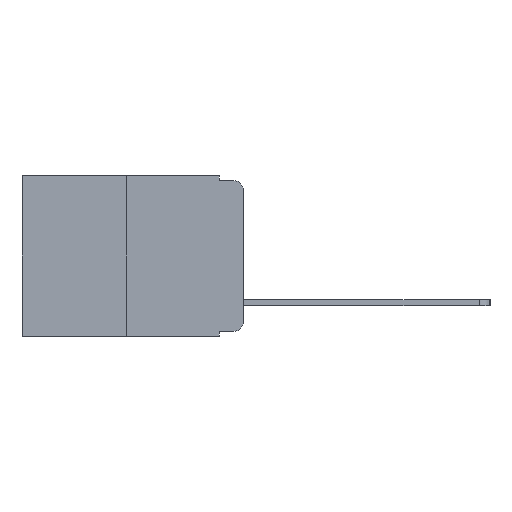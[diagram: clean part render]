
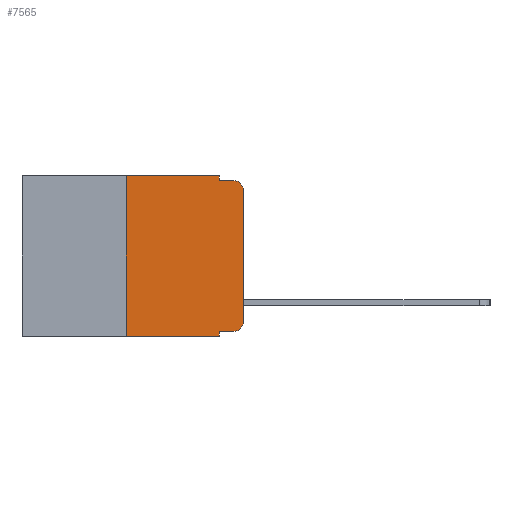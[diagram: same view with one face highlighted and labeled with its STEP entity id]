
A CAD part, left-side view. The second image highlights one B-rep face of the part: STEP entity #7565.
In plain terms, the highlighted planar face has unit normal (-1, 0, 0).
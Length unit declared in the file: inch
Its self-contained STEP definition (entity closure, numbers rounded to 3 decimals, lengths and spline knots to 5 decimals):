
#342 = PLANE ( 'NONE',  #7689 ) ;
#438 = CARTESIAN_POINT ( 'NONE',  ( 0., 0., -0.313 ) ) ;
#507 = LINE ( 'NONE', #7351, #3532 ) ;
#577 = CARTESIAN_POINT ( 'NONE',  ( 0., 0.02, -0.01 ) ) ;
#859 = LINE ( 'NONE', #7053, #8654 ) ;
#865 = CIRCLE ( 'NONE', #8322, 0.02 ) ;
#1341 = VERTEX_POINT ( 'NONE', #12617 ) ;
#1440 = LINE ( 'NONE', #11873, #6818 ) ;
#1530 = DIRECTION ( 'NONE',  ( 0., 0., -1. ) ) ;
#1536 = VERTEX_POINT ( 'NONE', #438 ) ;
#1583 = LINE ( 'NONE', #5567, #4167 ) ;
#1951 = CARTESIAN_POINT ( 'NONE',  ( 0., 0.25, 0. ) ) ;
#2065 = EDGE_CURVE ( 'NONE', #2365, #6524, #12882, .T. ) ;
#2129 = LINE ( 'NONE', #8547, #4656 ) ;
#2168 = DIRECTION ( 'NONE',  ( 0., 0., 1. ) ) ;
#2224 = EDGE_CURVE ( 'NONE', #4842, #2365, #507, .T. ) ;
#2331 = DIRECTION ( 'NONE',  ( -1., 0., 0. ) ) ;
#2365 = VERTEX_POINT ( 'NONE', #1951 ) ;
#2588 = CARTESIAN_POINT ( 'NONE',  ( 0., 0.02, -0.03 ) ) ;
#2692 = EDGE_CURVE ( 'NONE', #1341, #4808, #1440, .T. ) ;
#2743 = ORIENTED_EDGE ( 'NONE', *, *, #9179, .F. ) ;
#2858 = VERTEX_POINT ( 'NONE', #11105 ) ;
#3422 = EDGE_CURVE ( 'NONE', #11238, #4808, #865, .T. ) ;
#3443 = ORIENTED_EDGE ( 'NONE', *, *, #9512, .T. ) ;
#3532 = VECTOR ( 'NONE', #2168, 39.37008 ) ;
#3557 = CARTESIAN_POINT ( 'NONE',  ( 0., 0.051, -0.333 ) ) ;
#3721 = CARTESIAN_POINT ( 'NONE',  ( 0., 0.473, 0. ) ) ;
#3861 = CARTESIAN_POINT ( 'NONE',  ( 0., 0., -0.03 ) ) ;
#4126 = VECTOR ( 'NONE', #10918, 39.37008 ) ;
#4167 = VECTOR ( 'NONE', #11584, 39.37008 ) ;
#4443 = CARTESIAN_POINT ( 'NONE',  ( 0., 0.051, -0.333 ) ) ;
#4656 = VECTOR ( 'NONE', #9485, 39.37008 ) ;
#4731 = CARTESIAN_POINT ( 'NONE',  ( 0., 0.473, 0. ) ) ;
#4746 = CARTESIAN_POINT ( 'NONE',  ( 0., 0.051, 0. ) ) ;
#4758 = DIRECTION ( 'NONE',  ( 0., -1., 0. ) ) ;
#4808 = VERTEX_POINT ( 'NONE', #577 ) ;
#4842 = VERTEX_POINT ( 'NONE', #12291 ) ;
#4906 = CIRCLE ( 'NONE', #8618, 0.02 ) ;
#5273 = DIRECTION ( 'NONE',  ( 0., -1., 0. ) ) ;
#5285 = ORIENTED_EDGE ( 'NONE', *, *, #3422, .T. ) ;
#5567 = CARTESIAN_POINT ( 'NONE',  ( 0., 0.051, 0. ) ) ;
#5571 = EDGE_CURVE ( 'NONE', #1536, #11238, #6908, .T. ) ;
#6070 = DIRECTION ( 'NONE',  ( 0., -1., 0. ) ) ;
#6276 = ORIENTED_EDGE ( 'NONE', *, *, #12778, .F. ) ;
#6524 = VERTEX_POINT ( 'NONE', #4746 ) ;
#6807 = VECTOR ( 'NONE', #13489, 39.37008 ) ;
#6818 = VECTOR ( 'NONE', #5273, 39.37008 ) ;
#6908 = LINE ( 'NONE', #9965, #4126 ) ;
#7053 = CARTESIAN_POINT ( 'NONE',  ( 0., 0.473, -0.343 ) ) ;
#7121 = LINE ( 'NONE', #4443, #6807 ) ;
#7351 = CARTESIAN_POINT ( 'NONE',  ( 0., 0.25, 0. ) ) ;
#7423 = EDGE_CURVE ( 'NONE', #10950, #1536, #4906, .T. ) ;
#7565 = ADVANCED_FACE ( 'NONE', ( #8083 ), #342, .F. ) ;
#7689 = AXIS2_PLACEMENT_3D ( 'NONE', #3721, #7863, #1530 ) ;
#7863 = DIRECTION ( 'NONE',  ( 1., 0., 0. ) ) ;
#8083 = FACE_OUTER_BOUND ( 'NONE', #9638, .T. ) ;
#8322 = AXIS2_PLACEMENT_3D ( 'NONE', #2588, #12650, #12495 ) ;
#8493 = CARTESIAN_POINT ( 'NONE',  ( 0., 0.02, -0.333 ) ) ;
#8547 = CARTESIAN_POINT ( 'NONE',  ( 0., 0.051, 0. ) ) ;
#8582 = CARTESIAN_POINT ( 'NONE',  ( 0., 0.02, -0.313 ) ) ;
#8605 = ORIENTED_EDGE ( 'NONE', *, *, #2224, .F. ) ;
#8618 = AXIS2_PLACEMENT_3D ( 'NONE', #8582, #2331, #9564 ) ;
#8654 = VECTOR ( 'NONE', #6070, 39.37008 ) ;
#8901 = ORIENTED_EDGE ( 'NONE', *, *, #12132, .T. ) ;
#9179 = EDGE_CURVE ( 'NONE', #6524, #1341, #2129, .T. ) ;
#9485 = DIRECTION ( 'NONE',  ( 0., 0., -1. ) ) ;
#9512 = EDGE_CURVE ( 'NONE', #4842, #2858, #859, .T. ) ;
#9564 = DIRECTION ( 'NONE',  ( 0., 0., -1. ) ) ;
#9638 = EDGE_LOOP ( 'NONE', ( #10305, #5285, #10622, #2743, #10935, #8605, #3443, #6276, #8901, #11585 ) ) ;
#9965 = CARTESIAN_POINT ( 'NONE',  ( 0., 0., 0. ) ) ;
#10305 = ORIENTED_EDGE ( 'NONE', *, *, #5571, .T. ) ;
#10622 = ORIENTED_EDGE ( 'NONE', *, *, #2692, .F. ) ;
#10918 = DIRECTION ( 'NONE',  ( 0., 0., 1. ) ) ;
#10935 = ORIENTED_EDGE ( 'NONE', *, *, #2065, .F. ) ;
#10950 = VERTEX_POINT ( 'NONE', #8493 ) ;
#11105 = CARTESIAN_POINT ( 'NONE',  ( 0., 0.051, -0.343 ) ) ;
#11238 = VERTEX_POINT ( 'NONE', #3861 ) ;
#11584 = DIRECTION ( 'NONE',  ( 0., 0., -1. ) ) ;
#11585 = ORIENTED_EDGE ( 'NONE', *, *, #7423, .T. ) ;
#11608 = VERTEX_POINT ( 'NONE', #3557 ) ;
#11873 = CARTESIAN_POINT ( 'NONE',  ( 0., 0.051, -0.01 ) ) ;
#12132 = EDGE_CURVE ( 'NONE', #11608, #10950, #7121, .T. ) ;
#12291 = CARTESIAN_POINT ( 'NONE',  ( 0., 0.25, -0.343 ) ) ;
#12495 = DIRECTION ( 'NONE',  ( 0., 0., -1. ) ) ;
#12617 = CARTESIAN_POINT ( 'NONE',  ( 0., 0.051, -0.01 ) ) ;
#12650 = DIRECTION ( 'NONE',  ( -1., 0., 0. ) ) ;
#12778 = EDGE_CURVE ( 'NONE', #11608, #2858, #1583, .T. ) ;
#12882 = LINE ( 'NONE', #4731, #13177 ) ;
#13177 = VECTOR ( 'NONE', #4758, 39.37008 ) ;
#13489 = DIRECTION ( 'NONE',  ( 0., -1., 0. ) ) ;
